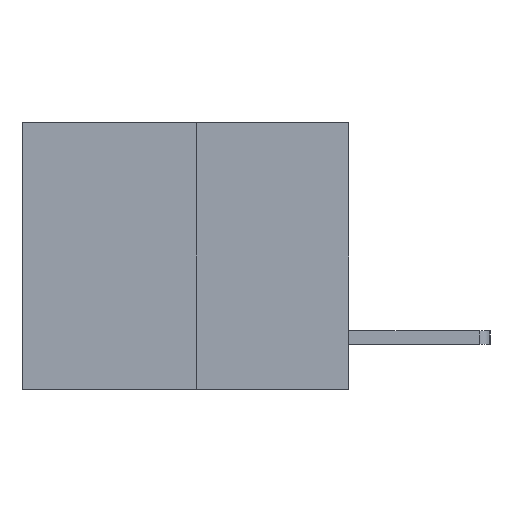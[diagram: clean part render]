
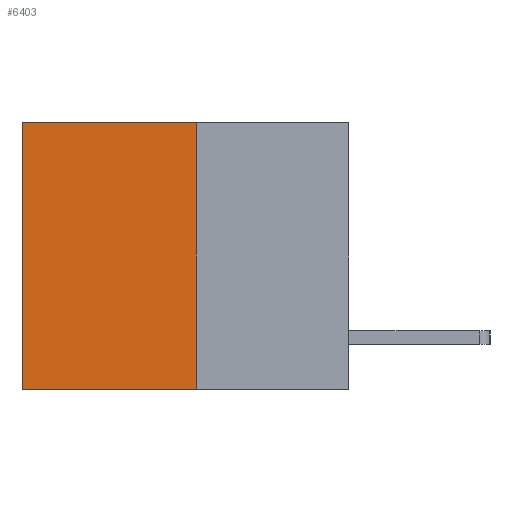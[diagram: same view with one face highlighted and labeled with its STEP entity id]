
A CAD part, left-side view. The second image highlights one B-rep face of the part: STEP entity #6403.
In plain terms, the highlighted planar face has unit normal (-1, 0, 0).
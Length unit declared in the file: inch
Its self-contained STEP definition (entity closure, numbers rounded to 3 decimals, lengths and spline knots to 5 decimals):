
#31 = VERTEX_POINT ( 'NONE', #1060 ) ;
#259 = VERTEX_POINT ( 'NONE', #7572 ) ;
#491 = LINE ( 'NONE', #4344, #1869 ) ;
#1060 = CARTESIAN_POINT ( 'NONE',  ( 0.3165, 0.6, -0.49 ) ) ;
#1376 = DIRECTION ( 'NONE',  ( 0., 1., 0. ) ) ;
#1543 = PLANE ( 'NONE',  #5926 ) ;
#1645 = CARTESIAN_POINT ( 'NONE',  ( 0.3165, 0.28, -0.49 ) ) ;
#1714 = VERTEX_POINT ( 'NONE', #1870 ) ;
#1738 = EDGE_CURVE ( 'NONE', #259, #31, #3541, .T. ) ;
#1869 = VECTOR ( 'NONE', #2303, 39.37008 ) ;
#1870 = CARTESIAN_POINT ( 'NONE',  ( 0.3165, 0.28, 0. ) ) ;
#1990 = VECTOR ( 'NONE', #1376, 39.37008 ) ;
#2303 = DIRECTION ( 'NONE',  ( 0., 1., 0. ) ) ;
#2705 = LINE ( 'NONE', #5085, #3555 ) ;
#3267 = CARTESIAN_POINT ( 'NONE',  ( 0.3165, 0.6, -0.49 ) ) ;
#3541 = LINE ( 'NONE', #3267, #5333 ) ;
#3555 = VECTOR ( 'NONE', #8461, 39.37008 ) ;
#3748 = FACE_OUTER_BOUND ( 'NONE', #5852, .T. ) ;
#4183 = CARTESIAN_POINT ( 'NONE',  ( 0.3165, 0.28, -0.49 ) ) ;
#4344 = CARTESIAN_POINT ( 'NONE',  ( 0.3165, 0.28, 0. ) ) ;
#4611 = EDGE_CURVE ( 'NONE', #6363, #31, #6428, .T. ) ;
#4719 = ORIENTED_EDGE ( 'NONE', *, *, #1738, .T. ) ;
#5004 = DIRECTION ( 'NONE',  ( 0., 0., -1. ) ) ;
#5085 = CARTESIAN_POINT ( 'NONE',  ( 0.3165, 0.28, -0.49 ) ) ;
#5324 = ORIENTED_EDGE ( 'NONE', *, *, #7647, .F. ) ;
#5333 = VECTOR ( 'NONE', #8008, 39.37008 ) ;
#5454 = EDGE_CURVE ( 'NONE', #1714, #259, #491, .T. ) ;
#5852 = EDGE_LOOP ( 'NONE', ( #4719, #7153, #5324, #8039 ) ) ;
#5926 = AXIS2_PLACEMENT_3D ( 'NONE', #1645, #6266, #5004 ) ;
#6266 = DIRECTION ( 'NONE',  ( 1., 0., 0. ) ) ;
#6363 = VERTEX_POINT ( 'NONE', #7628 ) ;
#6403 = ADVANCED_FACE ( 'NONE', ( #3748 ), #1543, .F. ) ;
#6428 = LINE ( 'NONE', #4183, #1990 ) ;
#7153 = ORIENTED_EDGE ( 'NONE', *, *, #4611, .F. ) ;
#7572 = CARTESIAN_POINT ( 'NONE',  ( 0.3165, 0.6, 0. ) ) ;
#7628 = CARTESIAN_POINT ( 'NONE',  ( 0.3165, 0.28, -0.49 ) ) ;
#7647 = EDGE_CURVE ( 'NONE', #1714, #6363, #2705, .T. ) ;
#8008 = DIRECTION ( 'NONE',  ( 0., 0., -1. ) ) ;
#8039 = ORIENTED_EDGE ( 'NONE', *, *, #5454, .T. ) ;
#8461 = DIRECTION ( 'NONE',  ( 0., 0., -1. ) ) ;
